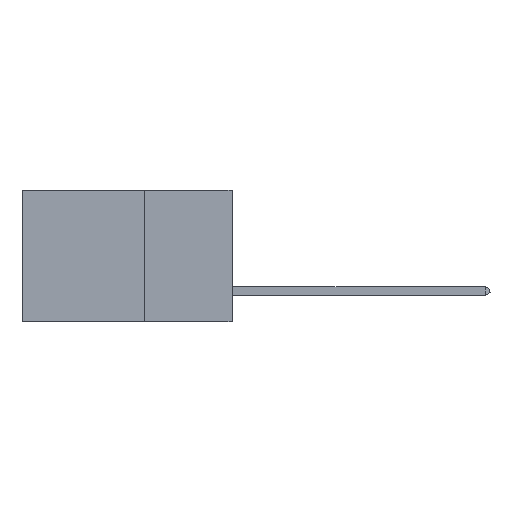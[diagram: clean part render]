
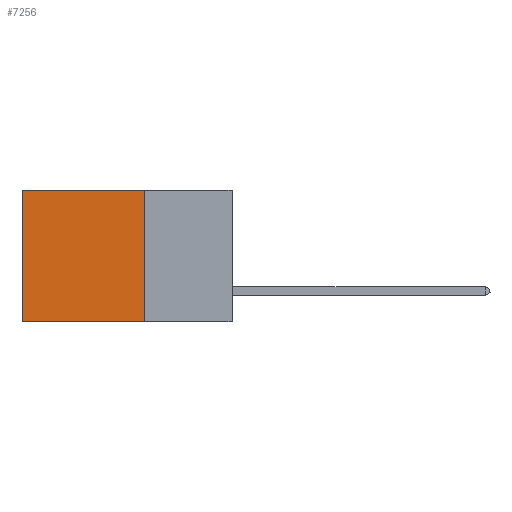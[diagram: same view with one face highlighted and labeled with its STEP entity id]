
A CAD part, left-side view. The second image highlights one B-rep face of the part: STEP entity #7256.
In plain terms, the highlighted planar face has unit normal (-1, 0, 0).
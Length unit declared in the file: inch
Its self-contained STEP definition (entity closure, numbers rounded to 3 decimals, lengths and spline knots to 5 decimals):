
#172 = VECTOR ( 'NONE', #1678, 39.37008 ) ;
#384 = FACE_OUTER_BOUND ( 'NONE', #1357, .T. ) ;
#606 = CARTESIAN_POINT ( 'NONE',  ( 0.2875, 0.25, -0.375 ) ) ;
#840 = DIRECTION ( 'NONE',  ( 0., 1., 0. ) ) ;
#1169 = VERTEX_POINT ( 'NONE', #5441 ) ;
#1357 = EDGE_LOOP ( 'NONE', ( #4659, #11634, #1618, #7152 ) ) ;
#1382 = CARTESIAN_POINT ( 'NONE',  ( 0.2875, 0.25, -0.375 ) ) ;
#1441 = VECTOR ( 'NONE', #1576, 39.37008 ) ;
#1576 = DIRECTION ( 'NONE',  ( 0., 0., -1. ) ) ;
#1618 = ORIENTED_EDGE ( 'NONE', *, *, #3195, .F. ) ;
#1678 = DIRECTION ( 'NONE',  ( 0., 1., 0. ) ) ;
#2449 = AXIS2_PLACEMENT_3D ( 'NONE', #5448, #12517, #7276 ) ;
#2557 = LINE ( 'NONE', #1382, #1441 ) ;
#3195 = EDGE_CURVE ( 'NONE', #11401, #4589, #2557, .T. ) ;
#3703 = CARTESIAN_POINT ( 'NONE',  ( 0.2875, 0.25, 0. ) ) ;
#3857 = LINE ( 'NONE', #11807, #9439 ) ;
#4589 = VERTEX_POINT ( 'NONE', #606 ) ;
#4659 = ORIENTED_EDGE ( 'NONE', *, *, #6158, .T. ) ;
#5317 = EDGE_CURVE ( 'NONE', #11401, #12281, #10732, .T. ) ;
#5441 = CARTESIAN_POINT ( 'NONE',  ( 0.2875, 0.6, -0.375 ) ) ;
#5448 = CARTESIAN_POINT ( 'NONE',  ( 0.2875, 0.25, -0.375 ) ) ;
#5720 = LINE ( 'NONE', #7547, #6269 ) ;
#6158 = EDGE_CURVE ( 'NONE', #12281, #1169, #5720, .T. ) ;
#6269 = VECTOR ( 'NONE', #7750, 39.37008 ) ;
#6406 = CARTESIAN_POINT ( 'NONE',  ( 0.2875, 0.6, 0. ) ) ;
#7152 = ORIENTED_EDGE ( 'NONE', *, *, #5317, .T. ) ;
#7256 = ADVANCED_FACE ( 'NONE', ( #384 ), #10300, .F. ) ;
#7276 = DIRECTION ( 'NONE',  ( 0., 0., -1. ) ) ;
#7290 = CARTESIAN_POINT ( 'NONE',  ( 0.2875, 0.25, 0. ) ) ;
#7547 = CARTESIAN_POINT ( 'NONE',  ( 0.2875, 0.6, -0.375 ) ) ;
#7750 = DIRECTION ( 'NONE',  ( 0., 0., -1. ) ) ;
#9439 = VECTOR ( 'NONE', #840, 39.37008 ) ;
#10300 = PLANE ( 'NONE',  #2449 ) ;
#10732 = LINE ( 'NONE', #3703, #172 ) ;
#11401 = VERTEX_POINT ( 'NONE', #7290 ) ;
#11634 = ORIENTED_EDGE ( 'NONE', *, *, #12073, .F. ) ;
#11807 = CARTESIAN_POINT ( 'NONE',  ( 0.2875, 0.25, -0.375 ) ) ;
#12073 = EDGE_CURVE ( 'NONE', #4589, #1169, #3857, .T. ) ;
#12281 = VERTEX_POINT ( 'NONE', #6406 ) ;
#12517 = DIRECTION ( 'NONE',  ( 1., 0., 0. ) ) ;
